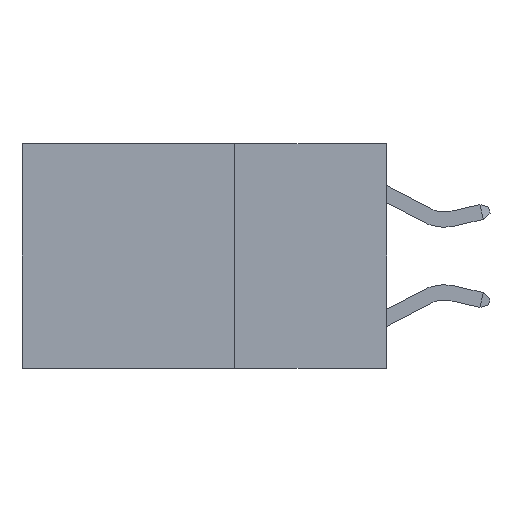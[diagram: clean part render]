
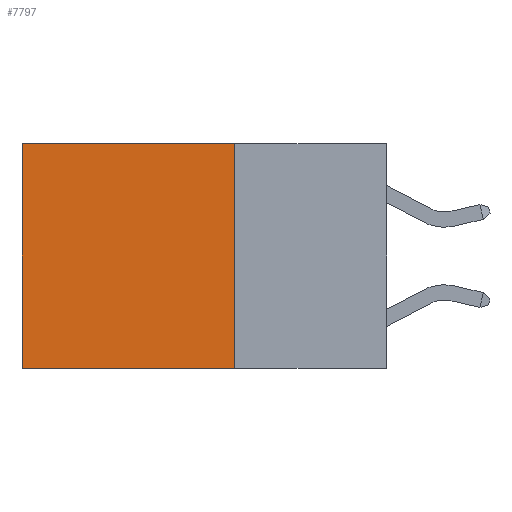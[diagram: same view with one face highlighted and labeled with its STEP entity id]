
A CAD part, left-side view. The second image highlights one B-rep face of the part: STEP entity #7797.
In plain terms, the highlighted planar face has unit normal (-1, 0, 0).
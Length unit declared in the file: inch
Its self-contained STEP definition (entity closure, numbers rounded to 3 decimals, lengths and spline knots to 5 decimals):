
#163 = PLANE ( 'NONE',  #2533 ) ;
#412 = CARTESIAN_POINT ( 'NONE',  ( 0.2625, 0.25, 0. ) ) ;
#1371 = LINE ( 'NONE', #7623, #3973 ) ;
#1495 = CARTESIAN_POINT ( 'NONE',  ( 0.2625, 0.25, 0. ) ) ;
#1519 = EDGE_CURVE ( 'NONE', #1943, #7530, #3913, .T. ) ;
#1730 = LINE ( 'NONE', #2286, #2277 ) ;
#1943 = VERTEX_POINT ( 'NONE', #1495 ) ;
#2277 = VECTOR ( 'NONE', #8406, 39.37008 ) ;
#2286 = CARTESIAN_POINT ( 'NONE',  ( 0.2625, 0.6, 0. ) ) ;
#2304 = CARTESIAN_POINT ( 'NONE',  ( 0.2625, 0.25, 0. ) ) ;
#2533 = AXIS2_PLACEMENT_3D ( 'NONE', #2304, #3714, #8565 ) ;
#2615 = ORIENTED_EDGE ( 'NONE', *, *, #6362, .T. ) ;
#3115 = LINE ( 'NONE', #4452, #7258 ) ;
#3299 = CARTESIAN_POINT ( 'NONE',  ( 0.2625, 0.25, -0.37 ) ) ;
#3372 = EDGE_CURVE ( 'NONE', #6505, #7775, #1730, .T. ) ;
#3655 = CARTESIAN_POINT ( 'NONE',  ( 0.2625, 0.6, -0.37 ) ) ;
#3714 = DIRECTION ( 'NONE',  ( 1., 0., 0. ) ) ;
#3848 = VECTOR ( 'NONE', #6735, 39.37008 ) ;
#3913 = LINE ( 'NONE', #412, #3848 ) ;
#3973 = VECTOR ( 'NONE', #4215, 39.37008 ) ;
#4215 = DIRECTION ( 'NONE',  ( 0., 1., 0. ) ) ;
#4375 = ORIENTED_EDGE ( 'NONE', *, *, #5943, .F. ) ;
#4452 = CARTESIAN_POINT ( 'NONE',  ( 0.2625, 0.25, -0.37 ) ) ;
#4492 = FACE_OUTER_BOUND ( 'NONE', #8863, .T. ) ;
#5943 = EDGE_CURVE ( 'NONE', #7530, #7775, #3115, .T. ) ;
#6150 = ORIENTED_EDGE ( 'NONE', *, *, #1519, .F. ) ;
#6245 = ORIENTED_EDGE ( 'NONE', *, *, #3372, .T. ) ;
#6362 = EDGE_CURVE ( 'NONE', #1943, #6505, #1371, .T. ) ;
#6505 = VERTEX_POINT ( 'NONE', #8426 ) ;
#6735 = DIRECTION ( 'NONE',  ( 0., 0., -1. ) ) ;
#7174 = DIRECTION ( 'NONE',  ( 0., 1., 0. ) ) ;
#7258 = VECTOR ( 'NONE', #7174, 39.37008 ) ;
#7530 = VERTEX_POINT ( 'NONE', #3299 ) ;
#7623 = CARTESIAN_POINT ( 'NONE',  ( 0.2625, 0.25, 0. ) ) ;
#7775 = VERTEX_POINT ( 'NONE', #3655 ) ;
#7797 = ADVANCED_FACE ( 'NONE', ( #4492 ), #163, .F. ) ;
#8406 = DIRECTION ( 'NONE',  ( 0., 0., -1. ) ) ;
#8426 = CARTESIAN_POINT ( 'NONE',  ( 0.2625, 0.6, 0. ) ) ;
#8565 = DIRECTION ( 'NONE',  ( 0., 0., -1. ) ) ;
#8863 = EDGE_LOOP ( 'NONE', ( #6245, #4375, #6150, #2615 ) ) ;
